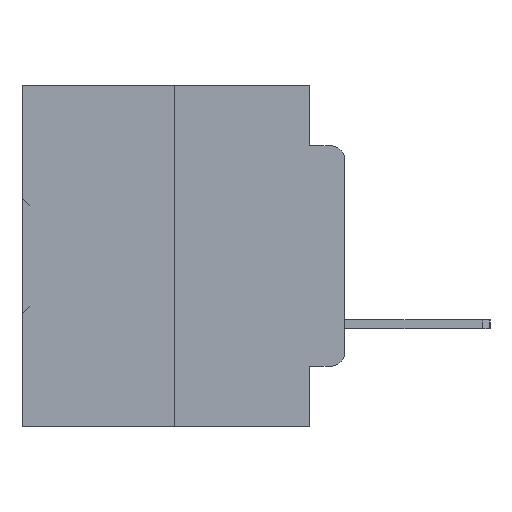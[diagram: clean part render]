
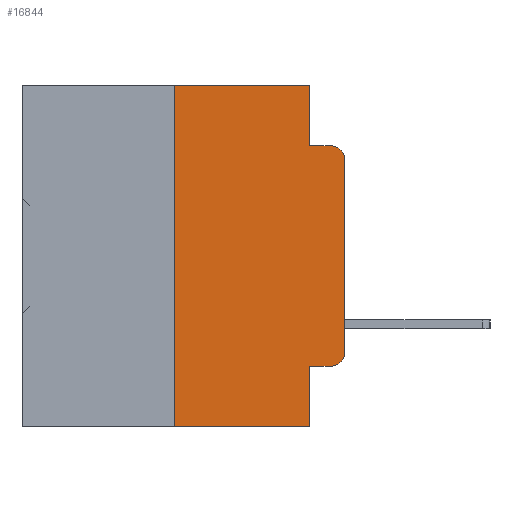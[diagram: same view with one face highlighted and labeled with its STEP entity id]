
A CAD part, left-side view. The second image highlights one B-rep face of the part: STEP entity #16844.
In plain terms, the highlighted planar face has unit normal (-1, 0, 0).
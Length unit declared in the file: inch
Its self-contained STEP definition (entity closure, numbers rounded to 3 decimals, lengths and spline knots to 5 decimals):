
#951 = EDGE_CURVE ( 'NONE', #22966, #11868, #7006, .T. ) ;
#1055 = VERTEX_POINT ( 'NONE', #18056 ) ;
#1913 = DIRECTION ( 'NONE',  ( -1., 0., 0. ) ) ;
#2037 = CARTESIAN_POINT ( 'NONE',  ( 0., 0.473, 0. ) ) ;
#2294 = CARTESIAN_POINT ( 'NONE',  ( 0., 0.473, -0.5 ) ) ;
#2342 = LINE ( 'NONE', #2294, #34212 ) ;
#2922 = EDGE_CURVE ( 'NONE', #11868, #1055, #28747, .T. ) ;
#2996 = DIRECTION ( 'NONE',  ( 0., 0., -1. ) ) ;
#3042 = VERTEX_POINT ( 'NONE', #24430 ) ;
#3082 = VERTEX_POINT ( 'NONE', #9991 ) ;
#3317 = CARTESIAN_POINT ( 'NONE',  ( 0., 0., -0.3915 ) ) ;
#3957 = PLANE ( 'NONE',  #4960 ) ;
#4295 = AXIS2_PLACEMENT_3D ( 'NONE', #16076, #36346, #19046 ) ;
#4885 = EDGE_CURVE ( 'NONE', #32351, #1055, #20412, .T. ) ;
#4960 = AXIS2_PLACEMENT_3D ( 'NONE', #24365, #9810, #30188 ) ;
#6397 = CARTESIAN_POINT ( 'NONE',  ( 0., 0.051, 0. ) ) ;
#7006 = LINE ( 'NONE', #23416, #22588 ) ;
#7331 = VECTOR ( 'NONE', #34100, 39.37008 ) ;
#7558 = EDGE_CURVE ( 'NONE', #3082, #17746, #35500, .T. ) ;
#7825 = DIRECTION ( 'NONE',  ( 0., 0., -1. ) ) ;
#8643 = DIRECTION ( 'NONE',  ( 0., -1., 0. ) ) ;
#8678 = VERTEX_POINT ( 'NONE', #33544 ) ;
#9247 = ORIENTED_EDGE ( 'NONE', *, *, #25197, .F. ) ;
#9662 = LINE ( 'NONE', #11458, #21566 ) ;
#9810 = DIRECTION ( 'NONE',  ( 1., 0., 0. ) ) ;
#9958 = VERTEX_POINT ( 'NONE', #33747 ) ;
#9991 = CARTESIAN_POINT ( 'NONE',  ( 0., 0.02, -0.4115 ) ) ;
#10566 = DIRECTION ( 'NONE',  ( 0., 0., 1. ) ) ;
#11218 = ORIENTED_EDGE ( 'NONE', *, *, #4885, .T. ) ;
#11458 = CARTESIAN_POINT ( 'NONE',  ( 0., 0.051, -0.4115 ) ) ;
#11868 = VERTEX_POINT ( 'NONE', #30977 ) ;
#12295 = ORIENTED_EDGE ( 'NONE', *, *, #951, .F. ) ;
#12300 = CARTESIAN_POINT ( 'NONE',  ( 0., 0.051, -0.0885 ) ) ;
#13329 = ORIENTED_EDGE ( 'NONE', *, *, #18569, .T. ) ;
#13656 = FACE_OUTER_BOUND ( 'NONE', #32805, .T. ) ;
#15049 = VECTOR ( 'NONE', #7825, 39.37008 ) ;
#15348 = EDGE_CURVE ( 'NONE', #8678, #3082, #9662, .T. ) ;
#16076 = CARTESIAN_POINT ( 'NONE',  ( 0., 0.02, -0.1085 ) ) ;
#16844 = ADVANCED_FACE ( 'NONE', ( #13656 ), #3957, .F. ) ;
#17205 = VERTEX_POINT ( 'NONE', #28891 ) ;
#17746 = VERTEX_POINT ( 'NONE', #3317 ) ;
#18056 = CARTESIAN_POINT ( 'NONE',  ( 0., 0.02, -0.0885 ) ) ;
#18249 = CARTESIAN_POINT ( 'NONE',  ( 0., 0., -0.1085 ) ) ;
#18456 = ORIENTED_EDGE ( 'NONE', *, *, #27111, .F. ) ;
#18492 = ORIENTED_EDGE ( 'NONE', *, *, #2922, .F. ) ;
#18569 = EDGE_CURVE ( 'NONE', #17746, #32351, #21836, .T. ) ;
#19046 = DIRECTION ( 'NONE',  ( 0., 0., -1. ) ) ;
#19412 = CARTESIAN_POINT ( 'NONE',  ( 0., 0.02, -0.3915 ) ) ;
#19796 = DIRECTION ( 'NONE',  ( 0., -1., 0. ) ) ;
#20412 = CIRCLE ( 'NONE', #4295, 0.02 ) ;
#21566 = VECTOR ( 'NONE', #8643, 39.37008 ) ;
#21836 = LINE ( 'NONE', #27351, #28632 ) ;
#22378 = DIRECTION ( 'NONE',  ( 0., 0., -1. ) ) ;
#22415 = CARTESIAN_POINT ( 'NONE',  ( 0., 0.051, 0. ) ) ;
#22588 = VECTOR ( 'NONE', #2996, 39.37008 ) ;
#22903 = LINE ( 'NONE', #2037, #7331 ) ;
#22966 = VERTEX_POINT ( 'NONE', #6397 ) ;
#23210 = AXIS2_PLACEMENT_3D ( 'NONE', #19412, #1913, #22378 ) ;
#23416 = CARTESIAN_POINT ( 'NONE',  ( 0., 0.051, 0. ) ) ;
#24030 = VECTOR ( 'NONE', #10566, 39.37008 ) ;
#24365 = CARTESIAN_POINT ( 'NONE',  ( 0., 0.473, 0. ) ) ;
#24430 = CARTESIAN_POINT ( 'NONE',  ( 0., 0.25, 0. ) ) ;
#25197 = EDGE_CURVE ( 'NONE', #8678, #9958, #30558, .T. ) ;
#27111 = EDGE_CURVE ( 'NONE', #17205, #3042, #30855, .T. ) ;
#27351 = CARTESIAN_POINT ( 'NONE',  ( 0., 0., 0. ) ) ;
#27971 = ORIENTED_EDGE ( 'NONE', *, *, #34451, .F. ) ;
#28018 = CARTESIAN_POINT ( 'NONE',  ( 0., 0.25, 0. ) ) ;
#28331 = ORIENTED_EDGE ( 'NONE', *, *, #30040, .T. ) ;
#28632 = VECTOR ( 'NONE', #30260, 39.37008 ) ;
#28747 = LINE ( 'NONE', #12300, #29645 ) ;
#28886 = ORIENTED_EDGE ( 'NONE', *, *, #7558, .T. ) ;
#28891 = CARTESIAN_POINT ( 'NONE',  ( 0., 0.25, -0.5 ) ) ;
#29645 = VECTOR ( 'NONE', #32663, 39.37008 ) ;
#30040 = EDGE_CURVE ( 'NONE', #17205, #9958, #2342, .T. ) ;
#30188 = DIRECTION ( 'NONE',  ( 0., 0., -1. ) ) ;
#30260 = DIRECTION ( 'NONE',  ( 0., 0., 1. ) ) ;
#30558 = LINE ( 'NONE', #22415, #15049 ) ;
#30855 = LINE ( 'NONE', #28018, #24030 ) ;
#30977 = CARTESIAN_POINT ( 'NONE',  ( 0., 0.051, -0.0885 ) ) ;
#32351 = VERTEX_POINT ( 'NONE', #18249 ) ;
#32663 = DIRECTION ( 'NONE',  ( 0., -1., 0. ) ) ;
#32805 = EDGE_LOOP ( 'NONE', ( #13329, #11218, #18492, #12295, #27971, #18456, #28331, #9247, #36378, #28886 ) ) ;
#33544 = CARTESIAN_POINT ( 'NONE',  ( 0., 0.051, -0.4115 ) ) ;
#33747 = CARTESIAN_POINT ( 'NONE',  ( 0., 0.051, -0.5 ) ) ;
#34100 = DIRECTION ( 'NONE',  ( 0., -1., 0. ) ) ;
#34212 = VECTOR ( 'NONE', #19796, 39.37008 ) ;
#34451 = EDGE_CURVE ( 'NONE', #3042, #22966, #22903, .T. ) ;
#35500 = CIRCLE ( 'NONE', #23210, 0.02 ) ;
#36346 = DIRECTION ( 'NONE',  ( -1., 0., 0. ) ) ;
#36378 = ORIENTED_EDGE ( 'NONE', *, *, #15348, .T. ) ;
